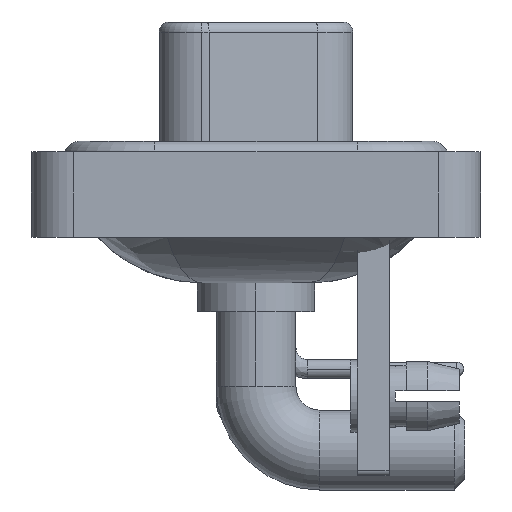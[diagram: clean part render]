
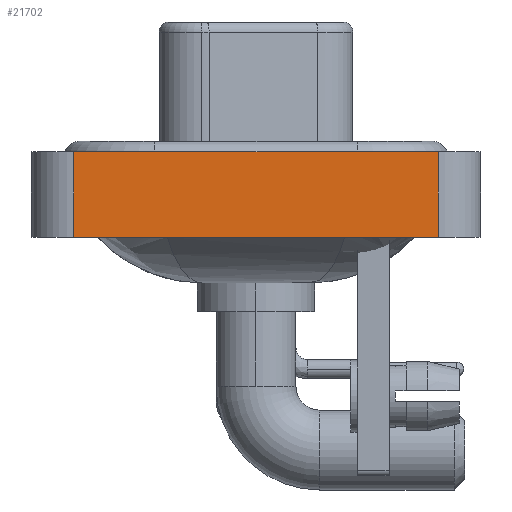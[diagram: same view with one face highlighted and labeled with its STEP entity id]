
A CAD part, left-side view. The second image highlights one B-rep face of the part: STEP entity #21702.
In plain terms, the highlighted planar face has unit normal (-1, 0, 0).
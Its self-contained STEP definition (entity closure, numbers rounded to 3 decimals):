
#735 = EDGE_LOOP ( 'NONE', ( #12406, #13291, #18904, #18433 ) ) ;
#2129 = CARTESIAN_POINT ( 'NONE',  ( -7.35, 8.55, -3.6 ) ) ;
#3386 = CARTESIAN_POINT ( 'NONE',  ( -7.35, -8.55, -3.6 ) ) ;
#3708 = CARTESIAN_POINT ( 'NONE',  ( -7.35, 8.55, -3.6 ) ) ;
#4356 = EDGE_CURVE ( 'NONE', #8959, #27141, #11905, .T. ) ;
#5453 = VERTEX_POINT ( 'NONE', #10916 ) ;
#5694 = VECTOR ( 'NONE', #7991, 1000. ) ;
#6648 = CARTESIAN_POINT ( 'NONE',  ( -7.35, 8.55, 0.4 ) ) ;
#7991 = DIRECTION ( 'NONE',  ( 0., -1., 0. ) ) ;
#8959 = VERTEX_POINT ( 'NONE', #3708 ) ;
#9888 = DIRECTION ( 'NONE',  ( 0., -1., 0. ) ) ;
#10463 = VERTEX_POINT ( 'NONE', #6648 ) ;
#10626 = CARTESIAN_POINT ( 'NONE',  ( -7.35, -8.55, -3.6 ) ) ;
#10769 = LINE ( 'NONE', #10626, #19172 ) ;
#10916 = CARTESIAN_POINT ( 'NONE',  ( -7.35, -8.55, 0.4 ) ) ;
#10946 = DIRECTION ( 'NONE',  ( 0., 0., 1. ) ) ;
#11905 = LINE ( 'NONE', #3386, #5694 ) ;
#12406 = ORIENTED_EDGE ( 'NONE', *, *, #14924, .T. ) ;
#13291 = ORIENTED_EDGE ( 'NONE', *, *, #27113, .F. ) ;
#13711 = VECTOR ( 'NONE', #10946, 1000. ) ;
#14279 = AXIS2_PLACEMENT_3D ( 'NONE', #21474, #23657, #27962 ) ;
#14924 = EDGE_CURVE ( 'NONE', #27141, #5453, #10769, .T. ) ;
#15541 = VECTOR ( 'NONE', #9888, 1000. ) ;
#17312 = PLANE ( 'NONE',  #14279 ) ;
#18433 = ORIENTED_EDGE ( 'NONE', *, *, #4356, .T. ) ;
#18550 = CARTESIAN_POINT ( 'NONE',  ( -7.35, -8.55, 0.4 ) ) ;
#18904 = ORIENTED_EDGE ( 'NONE', *, *, #19519, .F. ) ;
#19163 = FACE_OUTER_BOUND ( 'NONE', #735, .T. ) ;
#19172 = VECTOR ( 'NONE', #24318, 1000. ) ;
#19519 = EDGE_CURVE ( 'NONE', #8959, #10463, #26379, .T. ) ;
#20692 = LINE ( 'NONE', #18550, #15541 ) ;
#21474 = CARTESIAN_POINT ( 'NONE',  ( -7.35, -8.55, -3.6 ) ) ;
#21702 = ADVANCED_FACE ( 'NONE', ( #19163 ), #17312, .T. ) ;
#22588 = CARTESIAN_POINT ( 'NONE',  ( -7.35, -8.55, -3.6 ) ) ;
#23657 = DIRECTION ( 'NONE',  ( -1., 0., 0. ) ) ;
#24318 = DIRECTION ( 'NONE',  ( 0., 0., 1. ) ) ;
#26379 = LINE ( 'NONE', #2129, #13711 ) ;
#27113 = EDGE_CURVE ( 'NONE', #10463, #5453, #20692, .T. ) ;
#27141 = VERTEX_POINT ( 'NONE', #22588 ) ;
#27962 = DIRECTION ( 'NONE',  ( 0., 0., 1. ) ) ;
